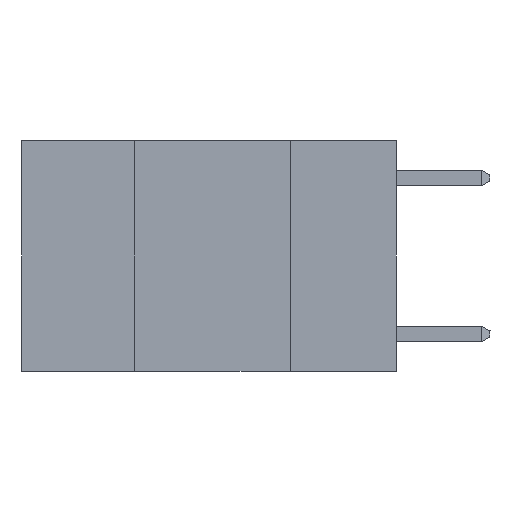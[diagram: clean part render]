
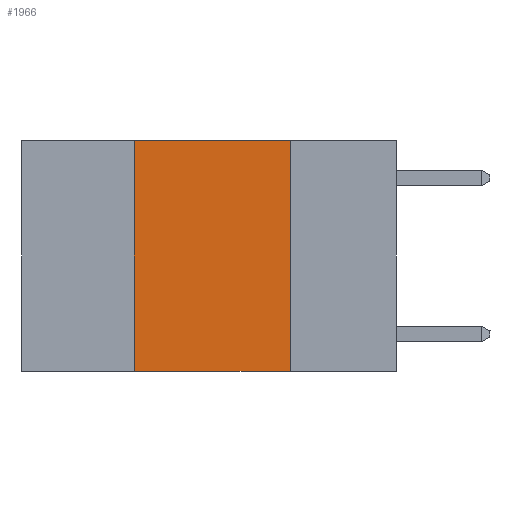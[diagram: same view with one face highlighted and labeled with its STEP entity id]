
A CAD part, left-side view. The second image highlights one B-rep face of the part: STEP entity #1966.
In plain terms, the highlighted planar face has unit normal (-1, 0, 0).
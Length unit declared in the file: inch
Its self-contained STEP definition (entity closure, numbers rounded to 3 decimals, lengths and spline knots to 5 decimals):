
#262 = EDGE_CURVE ( 'NONE', #5713, #6804, #1753, .T. ) ;
#549 = LINE ( 'NONE', #13667, #6471 ) ;
#681 = DIRECTION ( 'NONE',  ( 0., -1., 0. ) ) ;
#974 = EDGE_LOOP ( 'NONE', ( #10439, #1792, #4702, #7293 ) ) ;
#982 = FACE_OUTER_BOUND ( 'NONE', #974, .T. ) ;
#1753 = LINE ( 'NONE', #4311, #4330 ) ;
#1792 = ORIENTED_EDGE ( 'NONE', *, *, #10971, .F. ) ;
#1966 = ADVANCED_FACE ( 'NONE', ( #982 ), #8426, .F. ) ;
#2565 = EDGE_CURVE ( 'NONE', #9477, #12551, #6988, .T. ) ;
#2984 = CARTESIAN_POINT ( 'NONE',  ( 0., 0.6, 0. ) ) ;
#3302 = EDGE_CURVE ( 'NONE', #9477, #6804, #549, .T. ) ;
#4085 = DIRECTION ( 'NONE',  ( 0., 0., -1. ) ) ;
#4307 = CARTESIAN_POINT ( 'NONE',  ( 0., 0.42, -0.37 ) ) ;
#4311 = CARTESIAN_POINT ( 'NONE',  ( 0., 0.17, 0. ) ) ;
#4330 = VECTOR ( 'NONE', #7940, 39.37008 ) ;
#4702 = ORIENTED_EDGE ( 'NONE', *, *, #2565, .F. ) ;
#5713 = VERTEX_POINT ( 'NONE', #12097 ) ;
#6237 = DIRECTION ( 'NONE',  ( 0., 0., 1. ) ) ;
#6471 = VECTOR ( 'NONE', #681, 39.37008 ) ;
#6777 = VECTOR ( 'NONE', #6903, 39.37008 ) ;
#6804 = VERTEX_POINT ( 'NONE', #13664 ) ;
#6903 = DIRECTION ( 'NONE',  ( 0., -1., 0. ) ) ;
#6988 = LINE ( 'NONE', #9417, #7329 ) ;
#7293 = ORIENTED_EDGE ( 'NONE', *, *, #3302, .T. ) ;
#7329 = VECTOR ( 'NONE', #6237, 39.37008 ) ;
#7547 = AXIS2_PLACEMENT_3D ( 'NONE', #2984, #10546, #4085 ) ;
#7940 = DIRECTION ( 'NONE',  ( 0., 0., -1. ) ) ;
#8426 = PLANE ( 'NONE',  #7547 ) ;
#9417 = CARTESIAN_POINT ( 'NONE',  ( 0., 0.42, 0. ) ) ;
#9477 = VERTEX_POINT ( 'NONE', #4307 ) ;
#10439 = ORIENTED_EDGE ( 'NONE', *, *, #262, .F. ) ;
#10546 = DIRECTION ( 'NONE',  ( 1., 0., 0. ) ) ;
#10971 = EDGE_CURVE ( 'NONE', #12551, #5713, #13080, .T. ) ;
#12097 = CARTESIAN_POINT ( 'NONE',  ( 0., 0.17, 0. ) ) ;
#12278 = CARTESIAN_POINT ( 'NONE',  ( 0., 0.42, 0. ) ) ;
#12551 = VERTEX_POINT ( 'NONE', #12278 ) ;
#12941 = CARTESIAN_POINT ( 'NONE',  ( 0., 0.6, 0. ) ) ;
#13080 = LINE ( 'NONE', #12941, #6777 ) ;
#13664 = CARTESIAN_POINT ( 'NONE',  ( 0., 0.17, -0.37 ) ) ;
#13667 = CARTESIAN_POINT ( 'NONE',  ( 0., 0.6, -0.37 ) ) ;
